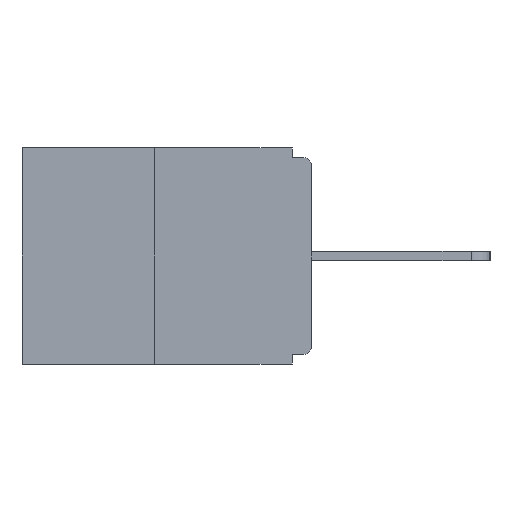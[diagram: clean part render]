
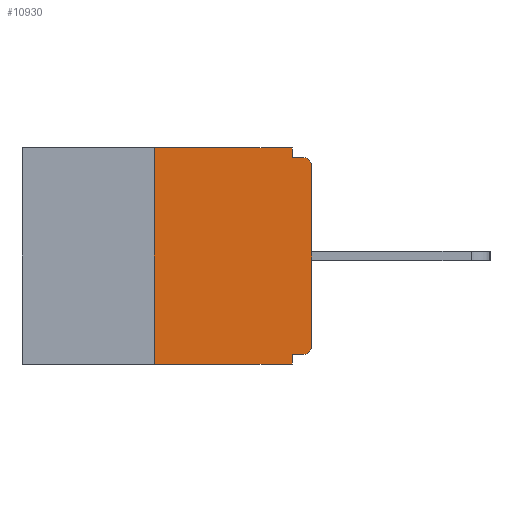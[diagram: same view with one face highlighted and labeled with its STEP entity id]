
A CAD part, left-side view. The second image highlights one B-rep face of the part: STEP entity #10930.
In plain terms, the highlighted planar face has unit normal (-1, 0, 0).
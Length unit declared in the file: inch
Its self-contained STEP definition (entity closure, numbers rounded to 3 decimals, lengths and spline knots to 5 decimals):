
#125 = ORIENTED_EDGE ( 'NONE', *, *, #6317, .T. ) ;
#691 = EDGE_CURVE ( 'NONE', #929, #20135, #7484, .T. ) ;
#929 = VERTEX_POINT ( 'NONE', #1360 ) ;
#1048 = CARTESIAN_POINT ( 'NONE',  ( 0., 0., -0.328 ) ) ;
#1246 = CARTESIAN_POINT ( 'NONE',  ( 0., 0.031, 0. ) ) ;
#1360 = CARTESIAN_POINT ( 'NONE',  ( 0., 0.015, -0.328 ) ) ;
#1772 = PLANE ( 'NONE',  #15294 ) ;
#1782 = CARTESIAN_POINT ( 'NONE',  ( 0., 0., -0.313 ) ) ;
#1894 = EDGE_CURVE ( 'NONE', #5753, #8535, #18798, .T. ) ;
#2349 = DIRECTION ( 'NONE',  ( 0., -1., 0. ) ) ;
#2635 = LINE ( 'NONE', #17277, #3620 ) ;
#2852 = DIRECTION ( 'NONE',  ( 0., 0., -1. ) ) ;
#2937 = AXIS2_PLACEMENT_3D ( 'NONE', #16886, #19741, #3717 ) ;
#3331 = VERTEX_POINT ( 'NONE', #10534 ) ;
#3402 = EDGE_CURVE ( 'NONE', #20135, #6705, #15494, .T. ) ;
#3453 = ORIENTED_EDGE ( 'NONE', *, *, #3402, .F. ) ;
#3620 = VECTOR ( 'NONE', #18642, 39.37008 ) ;
#3717 = DIRECTION ( 'NONE',  ( 0., 0., -1. ) ) ;
#3747 = ORIENTED_EDGE ( 'NONE', *, *, #9333, .T. ) ;
#4846 = DIRECTION ( 'NONE',  ( 1., 0., 0. ) ) ;
#5753 = VERTEX_POINT ( 'NONE', #20370 ) ;
#6031 = ORIENTED_EDGE ( 'NONE', *, *, #7003, .F. ) ;
#6317 = EDGE_CURVE ( 'NONE', #7323, #7192, #7963, .T. ) ;
#6705 = VERTEX_POINT ( 'NONE', #20839 ) ;
#7003 = EDGE_CURVE ( 'NONE', #8535, #18962, #16798, .T. ) ;
#7192 = VERTEX_POINT ( 'NONE', #8020 ) ;
#7323 = VERTEX_POINT ( 'NONE', #1782 ) ;
#7484 = LINE ( 'NONE', #1048, #14712 ) ;
#7487 = CARTESIAN_POINT ( 'NONE',  ( 0., 0.25, 0. ) ) ;
#7944 = VECTOR ( 'NONE', #2349, 39.37008 ) ;
#7963 = LINE ( 'NONE', #19376, #18028 ) ;
#8020 = CARTESIAN_POINT ( 'NONE',  ( 0., 0., -0.03 ) ) ;
#8099 = VECTOR ( 'NONE', #2852, 39.37008 ) ;
#8217 = DIRECTION ( 'NONE',  ( 0., 0., -1. ) ) ;
#8415 = VECTOR ( 'NONE', #9409, 39.37008 ) ;
#8535 = VERTEX_POINT ( 'NONE', #19516 ) ;
#9282 = EDGE_CURVE ( 'NONE', #929, #7323, #11672, .T. ) ;
#9333 = EDGE_CURVE ( 'NONE', #7192, #20193, #14026, .T. ) ;
#9409 = DIRECTION ( 'NONE',  ( 0., 0., 1. ) ) ;
#9687 = ORIENTED_EDGE ( 'NONE', *, *, #1894, .F. ) ;
#9877 = EDGE_CURVE ( 'NONE', #3331, #20193, #2635, .T. ) ;
#10534 = CARTESIAN_POINT ( 'NONE',  ( 0., 0.031, -0.015 ) ) ;
#10766 = DIRECTION ( 'NONE',  ( 0., 1., 0. ) ) ;
#10930 = ADVANCED_FACE ( 'NONE', ( #11285 ), #1772, .F. ) ;
#11285 = FACE_OUTER_BOUND ( 'NONE', #11674, .T. ) ;
#11672 = CIRCLE ( 'NONE', #2937, 0.015 ) ;
#11674 = EDGE_LOOP ( 'NONE', ( #6031, #9687, #13682, #3453, #14134, #16621, #125, #3747, #18771, #15075 ) ) ;
#12006 = VECTOR ( 'NONE', #14105, 39.37008 ) ;
#12122 = CARTESIAN_POINT ( 'NONE',  ( 0., 0.46, -0.343 ) ) ;
#13195 = DIRECTION ( 'NONE',  ( -1., 0., 0. ) ) ;
#13412 = CARTESIAN_POINT ( 'NONE',  ( 0., 0.46, 0. ) ) ;
#13495 = CARTESIAN_POINT ( 'NONE',  ( 0., 0.015, -0.03 ) ) ;
#13682 = ORIENTED_EDGE ( 'NONE', *, *, #19578, .T. ) ;
#14026 = CIRCLE ( 'NONE', #16403, 0.015 ) ;
#14105 = DIRECTION ( 'NONE',  ( 0., 0., -1. ) ) ;
#14134 = ORIENTED_EDGE ( 'NONE', *, *, #691, .F. ) ;
#14392 = DIRECTION ( 'NONE',  ( 0., 0., 1. ) ) ;
#14501 = EDGE_CURVE ( 'NONE', #18962, #3331, #15821, .T. ) ;
#14712 = VECTOR ( 'NONE', #10766, 39.37008 ) ;
#15075 = ORIENTED_EDGE ( 'NONE', *, *, #14501, .F. ) ;
#15096 = DIRECTION ( 'NONE',  ( 0., 0., -1. ) ) ;
#15270 = LINE ( 'NONE', #12122, #15727 ) ;
#15294 = AXIS2_PLACEMENT_3D ( 'NONE', #19321, #4846, #8217 ) ;
#15494 = LINE ( 'NONE', #18880, #8099 ) ;
#15727 = VECTOR ( 'NONE', #20247, 39.37008 ) ;
#15821 = LINE ( 'NONE', #1246, #12006 ) ;
#16403 = AXIS2_PLACEMENT_3D ( 'NONE', #13495, #13195, #15096 ) ;
#16621 = ORIENTED_EDGE ( 'NONE', *, *, #9282, .T. ) ;
#16798 = LINE ( 'NONE', #13412, #7944 ) ;
#16886 = CARTESIAN_POINT ( 'NONE',  ( 0., 0.015, -0.313 ) ) ;
#17277 = CARTESIAN_POINT ( 'NONE',  ( 0., 0., -0.015 ) ) ;
#17574 = CARTESIAN_POINT ( 'NONE',  ( 0., 0.015, -0.015 ) ) ;
#17671 = CARTESIAN_POINT ( 'NONE',  ( 0., 0.031, -0.328 ) ) ;
#18028 = VECTOR ( 'NONE', #14392, 39.37008 ) ;
#18642 = DIRECTION ( 'NONE',  ( 0., -1., 0. ) ) ;
#18771 = ORIENTED_EDGE ( 'NONE', *, *, #9877, .F. ) ;
#18798 = LINE ( 'NONE', #7487, #8415 ) ;
#18880 = CARTESIAN_POINT ( 'NONE',  ( 0., 0.031, -0.343 ) ) ;
#18962 = VERTEX_POINT ( 'NONE', #20852 ) ;
#19321 = CARTESIAN_POINT ( 'NONE',  ( 0., 0.46, 0. ) ) ;
#19376 = CARTESIAN_POINT ( 'NONE',  ( 0., 0., 0. ) ) ;
#19516 = CARTESIAN_POINT ( 'NONE',  ( 0., 0.25, 0. ) ) ;
#19578 = EDGE_CURVE ( 'NONE', #5753, #6705, #15270, .T. ) ;
#19741 = DIRECTION ( 'NONE',  ( -1., 0., 0. ) ) ;
#20135 = VERTEX_POINT ( 'NONE', #17671 ) ;
#20193 = VERTEX_POINT ( 'NONE', #17574 ) ;
#20247 = DIRECTION ( 'NONE',  ( 0., -1., 0. ) ) ;
#20370 = CARTESIAN_POINT ( 'NONE',  ( 0., 0.25, -0.343 ) ) ;
#20839 = CARTESIAN_POINT ( 'NONE',  ( 0., 0.031, -0.343 ) ) ;
#20852 = CARTESIAN_POINT ( 'NONE',  ( 0., 0.031, 0. ) ) ;
